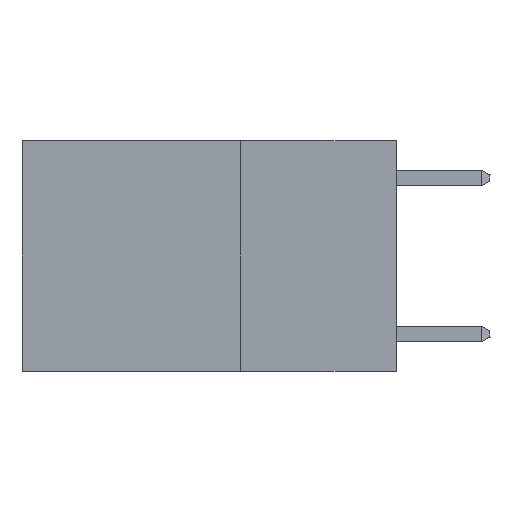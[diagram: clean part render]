
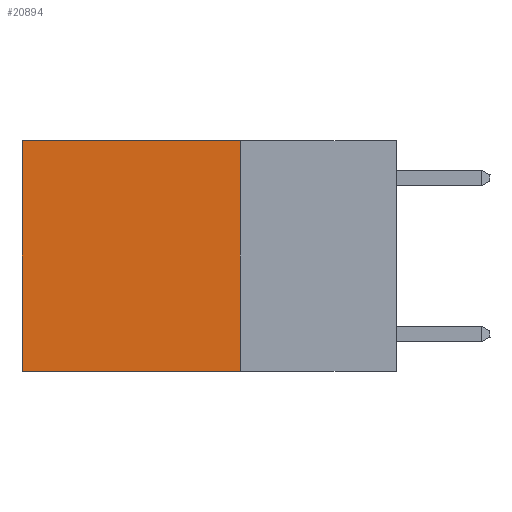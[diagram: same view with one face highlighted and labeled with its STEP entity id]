
A CAD part, left-side view. The second image highlights one B-rep face of the part: STEP entity #20894.
In plain terms, the highlighted planar face has unit normal (-1, 0, 0).
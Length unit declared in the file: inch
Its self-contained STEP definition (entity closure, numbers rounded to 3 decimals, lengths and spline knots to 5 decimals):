
#346 = CARTESIAN_POINT ( 'NONE',  ( 0.2625, 0.25, 0. ) ) ;
#405 = CARTESIAN_POINT ( 'NONE',  ( 0.2625, 0.6, -0.37 ) ) ;
#1325 = LINE ( 'NONE', #9574, #9914 ) ;
#1512 = ORIENTED_EDGE ( 'NONE', *, *, #14905, .F. ) ;
#2364 = ORIENTED_EDGE ( 'NONE', *, *, #18601, .F. ) ;
#2524 = DIRECTION ( 'NONE',  ( 0., 1., 0. ) ) ;
#3243 = AXIS2_PLACEMENT_3D ( 'NONE', #18446, #22334, #18069 ) ;
#4584 = EDGE_CURVE ( 'NONE', #7024, #20652, #1325, .T. ) ;
#5950 = PLANE ( 'NONE',  #3243 ) ;
#7024 = VERTEX_POINT ( 'NONE', #9101 ) ;
#7424 = VERTEX_POINT ( 'NONE', #18483 ) ;
#9101 = CARTESIAN_POINT ( 'NONE',  ( 0.2625, 0.6, 0. ) ) ;
#9574 = CARTESIAN_POINT ( 'NONE',  ( 0.2625, 0.6, 0. ) ) ;
#9914 = VECTOR ( 'NONE', #11063, 39.37008 ) ;
#9986 = ORIENTED_EDGE ( 'NONE', *, *, #4584, .T. ) ;
#10399 = FACE_OUTER_BOUND ( 'NONE', #18545, .T. ) ;
#10515 = LINE ( 'NONE', #346, #21787 ) ;
#10799 = LINE ( 'NONE', #15720, #20633 ) ;
#10934 = DIRECTION ( 'NONE',  ( 0., 1., 0. ) ) ;
#11063 = DIRECTION ( 'NONE',  ( 0., 0., -1. ) ) ;
#11637 = CARTESIAN_POINT ( 'NONE',  ( 0.2625, 0.25, 0. ) ) ;
#13103 = VERTEX_POINT ( 'NONE', #11637 ) ;
#14583 = VECTOR ( 'NONE', #14651, 39.37008 ) ;
#14651 = DIRECTION ( 'NONE',  ( 0., 0., -1. ) ) ;
#14905 = EDGE_CURVE ( 'NONE', #7424, #20652, #10799, .T. ) ;
#15720 = CARTESIAN_POINT ( 'NONE',  ( 0.2625, 0.25, -0.37 ) ) ;
#16413 = LINE ( 'NONE', #20928, #14583 ) ;
#18069 = DIRECTION ( 'NONE',  ( 0., 0., -1. ) ) ;
#18133 = EDGE_CURVE ( 'NONE', #13103, #7024, #10515, .T. ) ;
#18446 = CARTESIAN_POINT ( 'NONE',  ( 0.2625, 0.25, 0. ) ) ;
#18483 = CARTESIAN_POINT ( 'NONE',  ( 0.2625, 0.25, -0.37 ) ) ;
#18545 = EDGE_LOOP ( 'NONE', ( #9986, #1512, #2364, #19041 ) ) ;
#18601 = EDGE_CURVE ( 'NONE', #13103, #7424, #16413, .T. ) ;
#19041 = ORIENTED_EDGE ( 'NONE', *, *, #18133, .T. ) ;
#20633 = VECTOR ( 'NONE', #10934, 39.37008 ) ;
#20652 = VERTEX_POINT ( 'NONE', #405 ) ;
#20894 = ADVANCED_FACE ( 'NONE', ( #10399 ), #5950, .F. ) ;
#20928 = CARTESIAN_POINT ( 'NONE',  ( 0.2625, 0.25, 0. ) ) ;
#21787 = VECTOR ( 'NONE', #2524, 39.37008 ) ;
#22334 = DIRECTION ( 'NONE',  ( 1., 0., 0. ) ) ;
